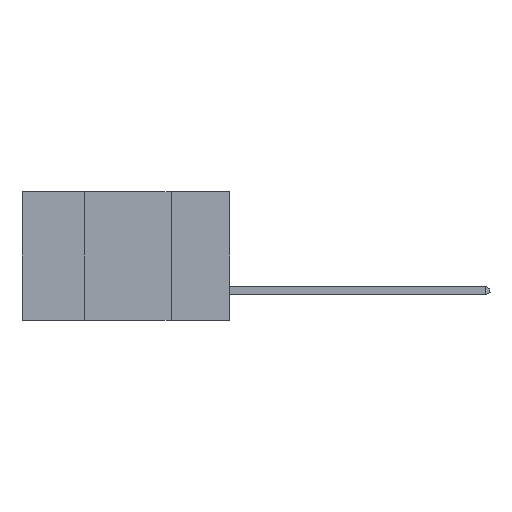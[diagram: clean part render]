
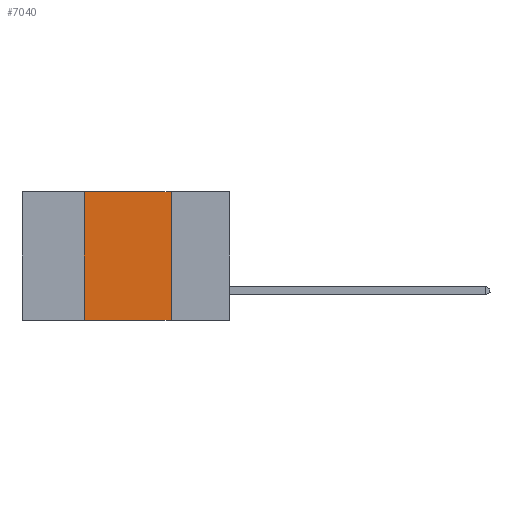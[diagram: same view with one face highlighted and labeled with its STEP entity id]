
A CAD part, left-side view. The second image highlights one B-rep face of the part: STEP entity #7040.
In plain terms, the highlighted planar face has unit normal (-1, 0, 0).
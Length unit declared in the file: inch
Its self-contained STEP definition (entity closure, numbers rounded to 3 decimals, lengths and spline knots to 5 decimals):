
#239 = EDGE_LOOP ( 'NONE', ( #9251, #459, #9150, #703 ) ) ;
#459 = ORIENTED_EDGE ( 'NONE', *, *, #7674, .F. ) ;
#481 = DIRECTION ( 'NONE',  ( 0., -1., 0. ) ) ;
#566 = EDGE_CURVE ( 'NONE', #4672, #8014, #2117, .T. ) ;
#604 = DIRECTION ( 'NONE',  ( 0., -1., 0. ) ) ;
#703 = ORIENTED_EDGE ( 'NONE', *, *, #1804, .T. ) ;
#836 = CARTESIAN_POINT ( 'NONE',  ( 0., 0.6, 0. ) ) ;
#1063 = CARTESIAN_POINT ( 'NONE',  ( 0., 0.42, 0. ) ) ;
#1098 = CARTESIAN_POINT ( 'NONE',  ( 0., 0.42, -0.37 ) ) ;
#1162 = EDGE_CURVE ( 'NONE', #5820, #7632, #5774, .T. ) ;
#1804 = EDGE_CURVE ( 'NONE', #5820, #8014, #4935, .T. ) ;
#2117 = LINE ( 'NONE', #7755, #6451 ) ;
#2287 = FACE_OUTER_BOUND ( 'NONE', #239, .T. ) ;
#2348 = DIRECTION ( 'NONE',  ( 1., 0., 0. ) ) ;
#2674 = VECTOR ( 'NONE', #2752, 39.37008 ) ;
#2752 = DIRECTION ( 'NONE',  ( 0., 0., 1. ) ) ;
#3122 = LINE ( 'NONE', #4752, #8920 ) ;
#4113 = CARTESIAN_POINT ( 'NONE',  ( 0., 0.42, 0. ) ) ;
#4436 = DIRECTION ( 'NONE',  ( 0., 0., -1. ) ) ;
#4672 = VERTEX_POINT ( 'NONE', #5856 ) ;
#4752 = CARTESIAN_POINT ( 'NONE',  ( 0., 0.6, 0. ) ) ;
#4935 = LINE ( 'NONE', #5443, #8294 ) ;
#5443 = CARTESIAN_POINT ( 'NONE',  ( 0., 0.6, -0.37 ) ) ;
#5553 = DIRECTION ( 'NONE',  ( 0., 0., -1. ) ) ;
#5774 = LINE ( 'NONE', #4113, #2674 ) ;
#5820 = VERTEX_POINT ( 'NONE', #1098 ) ;
#5856 = CARTESIAN_POINT ( 'NONE',  ( 0., 0.17, 0. ) ) ;
#6451 = VECTOR ( 'NONE', #5553, 39.37008 ) ;
#7040 = ADVANCED_FACE ( 'NONE', ( #2287 ), #8706, .F. ) ;
#7632 = VERTEX_POINT ( 'NONE', #1063 ) ;
#7674 = EDGE_CURVE ( 'NONE', #7632, #4672, #3122, .T. ) ;
#7755 = CARTESIAN_POINT ( 'NONE',  ( 0., 0.17, 0. ) ) ;
#8014 = VERTEX_POINT ( 'NONE', #8655 ) ;
#8294 = VECTOR ( 'NONE', #604, 39.37008 ) ;
#8655 = CARTESIAN_POINT ( 'NONE',  ( 0., 0.17, -0.37 ) ) ;
#8706 = PLANE ( 'NONE',  #8926 ) ;
#8920 = VECTOR ( 'NONE', #481, 39.37008 ) ;
#8926 = AXIS2_PLACEMENT_3D ( 'NONE', #836, #2348, #4436 ) ;
#9150 = ORIENTED_EDGE ( 'NONE', *, *, #1162, .F. ) ;
#9251 = ORIENTED_EDGE ( 'NONE', *, *, #566, .F. ) ;
